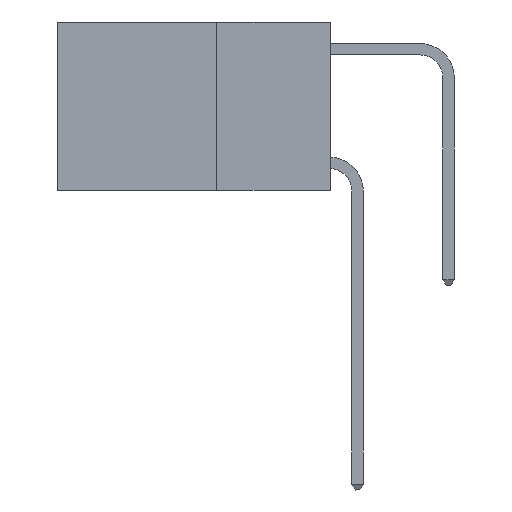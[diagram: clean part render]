
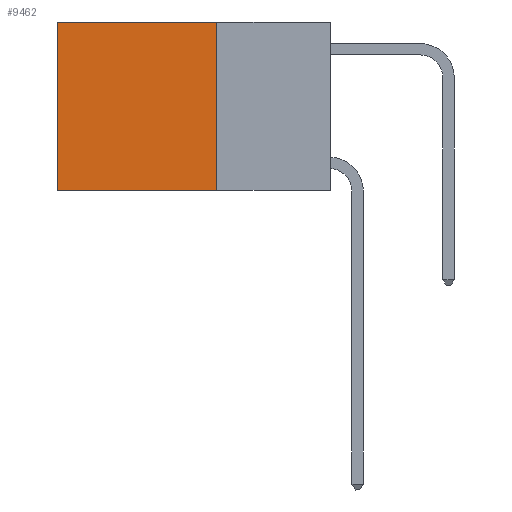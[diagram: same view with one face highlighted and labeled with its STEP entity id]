
A CAD part, left-side view. The second image highlights one B-rep face of the part: STEP entity #9462.
In plain terms, the highlighted planar face has unit normal (-1, 0, 0).
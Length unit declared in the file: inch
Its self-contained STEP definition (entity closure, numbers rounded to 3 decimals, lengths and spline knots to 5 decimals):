
#602 = LINE ( 'NONE', #13255, #4089 ) ;
#894 = DIRECTION ( 'NONE',  ( 0., 1., 0. ) ) ;
#1393 = EDGE_LOOP ( 'NONE', ( #12716, #9632, #7973, #6132 ) ) ;
#1788 = LINE ( 'NONE', #9858, #9426 ) ;
#2769 = CARTESIAN_POINT ( 'NONE',  ( 0.2625, 0.25, -0.37 ) ) ;
#2816 = LINE ( 'NONE', #7481, #4808 ) ;
#3238 = VERTEX_POINT ( 'NONE', #10980 ) ;
#3929 = CARTESIAN_POINT ( 'NONE',  ( 0.2625, 0.25, 0. ) ) ;
#4089 = VECTOR ( 'NONE', #8602, 39.37008 ) ;
#4172 = EDGE_CURVE ( 'NONE', #11010, #3238, #602, .T. ) ;
#4276 = DIRECTION ( 'NONE',  ( 1., 0., 0. ) ) ;
#4417 = CARTESIAN_POINT ( 'NONE',  ( 0.2625, 0.25, 0. ) ) ;
#4549 = EDGE_CURVE ( 'NONE', #7006, #11010, #2816, .T. ) ;
#4808 = VECTOR ( 'NONE', #12972, 39.37008 ) ;
#5421 = AXIS2_PLACEMENT_3D ( 'NONE', #4417, #4276, #11082 ) ;
#6132 = ORIENTED_EDGE ( 'NONE', *, *, #14125, .T. ) ;
#6559 = CARTESIAN_POINT ( 'NONE',  ( 0.2625, 0.6, 0. ) ) ;
#6563 = PLANE ( 'NONE',  #5421 ) ;
#7006 = VERTEX_POINT ( 'NONE', #3929 ) ;
#7481 = CARTESIAN_POINT ( 'NONE',  ( 0.2625, 0.25, 0. ) ) ;
#7973 = ORIENTED_EDGE ( 'NONE', *, *, #4549, .F. ) ;
#7977 = FACE_OUTER_BOUND ( 'NONE', #1393, .T. ) ;
#8063 = VECTOR ( 'NONE', #12840, 39.37008 ) ;
#8159 = VERTEX_POINT ( 'NONE', #6559 ) ;
#8602 = DIRECTION ( 'NONE',  ( 0., 1., 0. ) ) ;
#9426 = VECTOR ( 'NONE', #894, 39.37008 ) ;
#9462 = ADVANCED_FACE ( 'NONE', ( #7977 ), #6563, .F. ) ;
#9632 = ORIENTED_EDGE ( 'NONE', *, *, #4172, .F. ) ;
#9858 = CARTESIAN_POINT ( 'NONE',  ( 0.2625, 0.25, 0. ) ) ;
#10980 = CARTESIAN_POINT ( 'NONE',  ( 0.2625, 0.6, -0.37 ) ) ;
#11010 = VERTEX_POINT ( 'NONE', #2769 ) ;
#11082 = DIRECTION ( 'NONE',  ( 0., 0., -1. ) ) ;
#11514 = LINE ( 'NONE', #11591, #8063 ) ;
#11591 = CARTESIAN_POINT ( 'NONE',  ( 0.2625, 0.6, 0. ) ) ;
#12716 = ORIENTED_EDGE ( 'NONE', *, *, #14547, .T. ) ;
#12840 = DIRECTION ( 'NONE',  ( 0., 0., -1. ) ) ;
#12972 = DIRECTION ( 'NONE',  ( 0., 0., -1. ) ) ;
#13255 = CARTESIAN_POINT ( 'NONE',  ( 0.2625, 0.25, -0.37 ) ) ;
#14125 = EDGE_CURVE ( 'NONE', #7006, #8159, #1788, .T. ) ;
#14547 = EDGE_CURVE ( 'NONE', #8159, #3238, #11514, .T. ) ;
